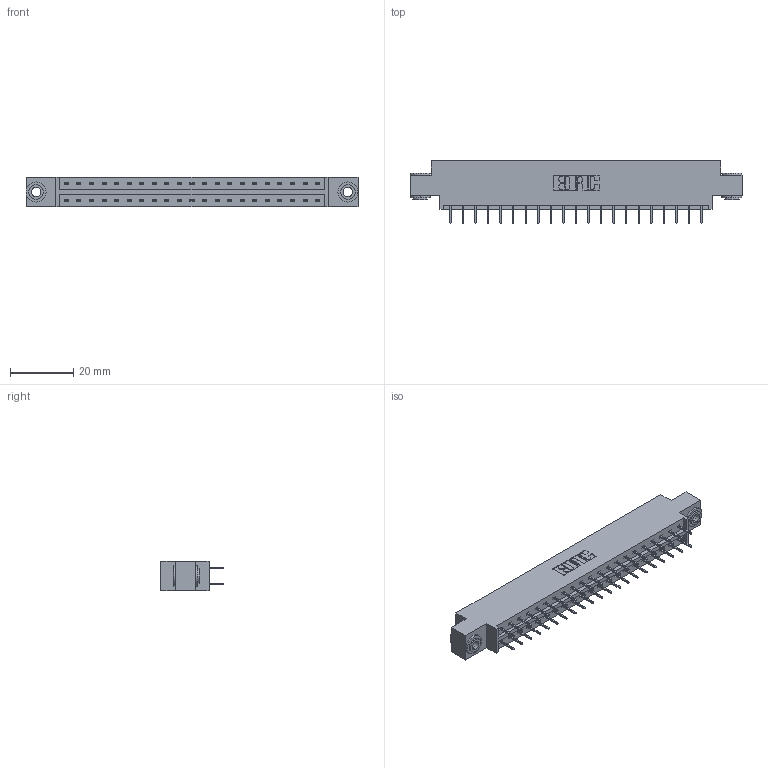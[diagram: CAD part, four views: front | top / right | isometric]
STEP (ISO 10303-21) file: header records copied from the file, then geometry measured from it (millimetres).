
FILE_DESCRIPTION (( 'STEP AP203' ), '1' );
FILE_NAME ('333-042-524-803.STEP', '2018-08-03T18:46:34', ( '' ), ( '' ), 'SwSTEP 2.0', 'SolidWorks 2016', '' );
FILE_SCHEMA (( 'CONFIG_CONTROL_DESIGN' ));
Length unit declared in the file: inch
Products named in the file (4): 345-292-001_345-293-124; 345-250-002_345-250-002-102; 333-042-524-803; 333 Part_Offset - .156 Dia - TH
Assembly tree (45 placements, depth 2):
  333-042-524-803
    333 Part_Offset - .156 Dia - TH
    345-292-001_345-293-124  x42
    345-250-002_345-250-002-102  x2
Bounding box: 104.75 x 19.69 x 9.4 mm (x, y, z)
Volume: 10226 mm3; surface area: 12115 mm2
Topology: 45 solids, 45 shells, 2508 faces, 7077 edges, 4546 vertices
Faces by surface type: plane 1848, cylinder 652, cone 8
Entity records: 17082 total; most frequent: CARTESIAN_POINT 2833, ORIENTED_EDGE 2762, DIRECTION 2491, EDGE_CURVE 1381, VECTOR 1233, LINE 1233, VERTEX_POINT 914, AXIS2_PLACEMENT_3D 629
